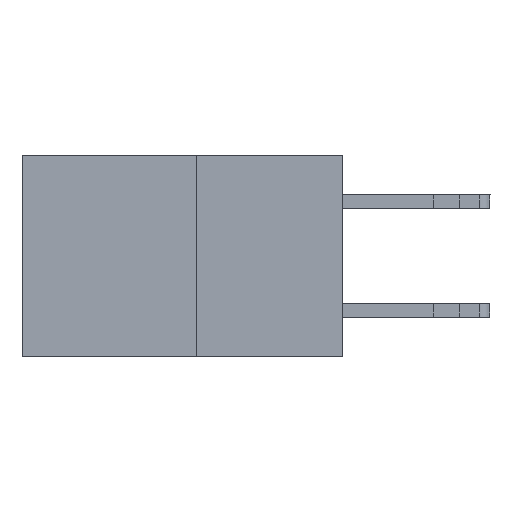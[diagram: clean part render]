
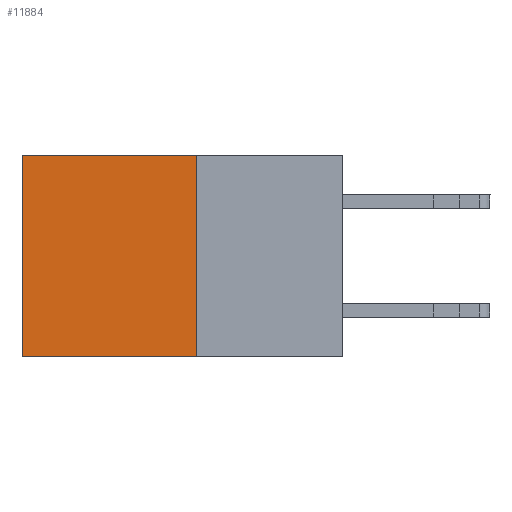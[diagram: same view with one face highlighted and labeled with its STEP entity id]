
A CAD part, left-side view. The second image highlights one B-rep face of the part: STEP entity #11884.
In plain terms, the highlighted planar face has unit normal (-1, 0, 0).
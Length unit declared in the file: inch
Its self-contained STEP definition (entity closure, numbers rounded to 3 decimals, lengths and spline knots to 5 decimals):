
#101 = VERTEX_POINT ( 'NONE', #22531 ) ;
#2346 = EDGE_CURVE ( 'NONE', #101, #24978, #13012, .T. ) ;
#3624 = DIRECTION ( 'NONE',  ( 0., 0., -1. ) ) ;
#4250 = CARTESIAN_POINT ( 'NONE',  ( 0.277, 0.59, -0.37 ) ) ;
#4655 = ORIENTED_EDGE ( 'NONE', *, *, #2346, .T. ) ;
#5036 = VERTEX_POINT ( 'NONE', #4250 ) ;
#5077 = EDGE_CURVE ( 'NONE', #18070, #5036, #9409, .T. ) ;
#5698 = LINE ( 'NONE', #14393, #22114 ) ;
#5832 = FACE_OUTER_BOUND ( 'NONE', #22022, .T. ) ;
#6048 = CARTESIAN_POINT ( 'NONE',  ( 0.277, 0.59, 0. ) ) ;
#7344 = DIRECTION ( 'NONE',  ( 0., 1., 0. ) ) ;
#7446 = ORIENTED_EDGE ( 'NONE', *, *, #5077, .F. ) ;
#8744 = DIRECTION ( 'NONE',  ( 0., 1., 0. ) ) ;
#9409 = LINE ( 'NONE', #18516, #22065 ) ;
#11884 = ADVANCED_FACE ( 'NONE', ( #5832 ), #17150, .F. ) ;
#12312 = VECTOR ( 'NONE', #8744, 39.37008 ) ;
#13012 = LINE ( 'NONE', #24326, #12312 ) ;
#14393 = CARTESIAN_POINT ( 'NONE',  ( 0.277, 0.59, -0.37 ) ) ;
#14607 = VECTOR ( 'NONE', #28509, 39.37008 ) ;
#14842 = CARTESIAN_POINT ( 'NONE',  ( 0.277, 0.27, -0.37 ) ) ;
#16095 = EDGE_CURVE ( 'NONE', #24978, #5036, #5698, .T. ) ;
#16235 = EDGE_CURVE ( 'NONE', #101, #18070, #28642, .T. ) ;
#16586 = AXIS2_PLACEMENT_3D ( 'NONE', #18777, #21125, #3624 ) ;
#17150 = PLANE ( 'NONE',  #16586 ) ;
#18070 = VERTEX_POINT ( 'NONE', #14842 ) ;
#18516 = CARTESIAN_POINT ( 'NONE',  ( 0.277, 0.27, -0.37 ) ) ;
#18777 = CARTESIAN_POINT ( 'NONE',  ( 0.277, 0.27, -0.37 ) ) ;
#21125 = DIRECTION ( 'NONE',  ( 1., 0., 0. ) ) ;
#21245 = ORIENTED_EDGE ( 'NONE', *, *, #16235, .F. ) ;
#21870 = CARTESIAN_POINT ( 'NONE',  ( 0.277, 0.27, -0.37 ) ) ;
#22022 = EDGE_LOOP ( 'NONE', ( #24311, #7446, #21245, #4655 ) ) ;
#22065 = VECTOR ( 'NONE', #7344, 39.37008 ) ;
#22114 = VECTOR ( 'NONE', #23359, 39.37008 ) ;
#22531 = CARTESIAN_POINT ( 'NONE',  ( 0.277, 0.27, 0. ) ) ;
#23359 = DIRECTION ( 'NONE',  ( 0., 0., -1. ) ) ;
#24311 = ORIENTED_EDGE ( 'NONE', *, *, #16095, .T. ) ;
#24326 = CARTESIAN_POINT ( 'NONE',  ( 0.277, 0.27, 0. ) ) ;
#24978 = VERTEX_POINT ( 'NONE', #6048 ) ;
#28509 = DIRECTION ( 'NONE',  ( 0., 0., -1. ) ) ;
#28642 = LINE ( 'NONE', #21870, #14607 ) ;
